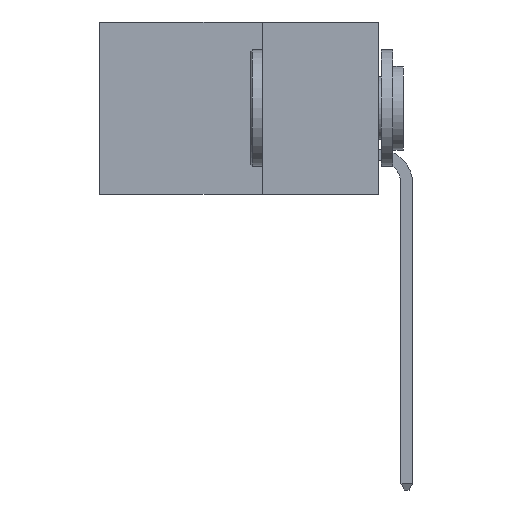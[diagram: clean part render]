
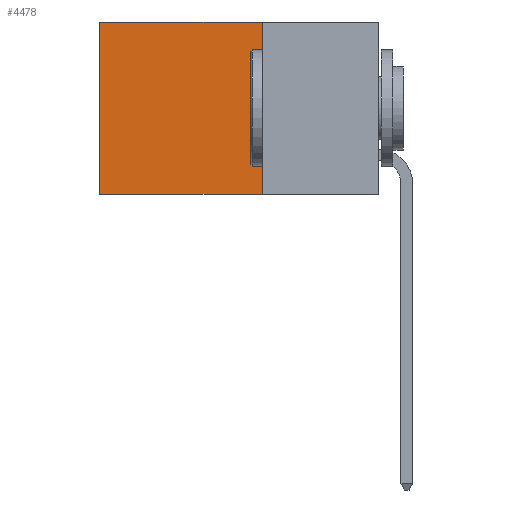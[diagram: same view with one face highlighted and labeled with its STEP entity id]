
A CAD part, left-side view. The second image highlights one B-rep face of the part: STEP entity #4478.
In plain terms, the highlighted planar face has unit normal (-1, 0, 0).
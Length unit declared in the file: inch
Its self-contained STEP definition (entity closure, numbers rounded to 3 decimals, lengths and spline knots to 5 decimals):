
#2251 = EDGE_CURVE ( 'NONE', #13459, #15585, #3702, .T. ) ;
#2489 = LINE ( 'NONE', #6536, #6465 ) ;
#3702 = LINE ( 'NONE', #6270, #20454 ) ;
#4478 = ADVANCED_FACE ( 'NONE', ( #19866 ), #14140, .F. ) ;
#5267 = DIRECTION ( 'NONE',  ( 0., 0., -1. ) ) ;
#6270 = CARTESIAN_POINT ( 'NONE',  ( 0.2615, 0.25, -0.37 ) ) ;
#6465 = VECTOR ( 'NONE', #5267, 39.37008 ) ;
#6536 = CARTESIAN_POINT ( 'NONE',  ( 0.2615, 0.6, -0.37 ) ) ;
#7289 = CARTESIAN_POINT ( 'NONE',  ( 0.2615, 0.6, -0.37 ) ) ;
#7563 = DIRECTION ( 'NONE',  ( 0., 1., 0. ) ) ;
#7832 = ORIENTED_EDGE ( 'NONE', *, *, #8437, .F. ) ;
#8437 = EDGE_CURVE ( 'NONE', #11577, #13459, #15739, .T. ) ;
#8834 = EDGE_CURVE ( 'NONE', #11577, #19460, #11801, .T. ) ;
#9093 = EDGE_CURVE ( 'NONE', #19460, #15585, #2489, .T. ) ;
#10314 = CARTESIAN_POINT ( 'NONE',  ( 0.2615, 0.25, -0.37 ) ) ;
#10750 = VECTOR ( 'NONE', #20789, 39.37008 ) ;
#11440 = DIRECTION ( 'NONE',  ( 0., 1., 0. ) ) ;
#11494 = CARTESIAN_POINT ( 'NONE',  ( 0.2615, 0.25, 0. ) ) ;
#11562 = ORIENTED_EDGE ( 'NONE', *, *, #8834, .T. ) ;
#11577 = VERTEX_POINT ( 'NONE', #13075 ) ;
#11801 = LINE ( 'NONE', #11494, #12315 ) ;
#12047 = ORIENTED_EDGE ( 'NONE', *, *, #9093, .T. ) ;
#12315 = VECTOR ( 'NONE', #11440, 39.37008 ) ;
#13075 = CARTESIAN_POINT ( 'NONE',  ( 0.2615, 0.25, 0. ) ) ;
#13459 = VERTEX_POINT ( 'NONE', #10314 ) ;
#13947 = DIRECTION ( 'NONE',  ( 0., 0., -1. ) ) ;
#13950 = DIRECTION ( 'NONE',  ( 1., 0., 0. ) ) ;
#14037 = EDGE_LOOP ( 'NONE', ( #12047, #17597, #7832, #11562 ) ) ;
#14140 = PLANE ( 'NONE',  #18800 ) ;
#14210 = CARTESIAN_POINT ( 'NONE',  ( 0.2615, 0.25, -0.37 ) ) ;
#15585 = VERTEX_POINT ( 'NONE', #7289 ) ;
#15739 = LINE ( 'NONE', #21401, #10750 ) ;
#17597 = ORIENTED_EDGE ( 'NONE', *, *, #2251, .F. ) ;
#18800 = AXIS2_PLACEMENT_3D ( 'NONE', #14210, #13950, #13947 ) ;
#19460 = VERTEX_POINT ( 'NONE', #21373 ) ;
#19866 = FACE_OUTER_BOUND ( 'NONE', #14037, .T. ) ;
#20454 = VECTOR ( 'NONE', #7563, 39.37008 ) ;
#20789 = DIRECTION ( 'NONE',  ( 0., 0., -1. ) ) ;
#21373 = CARTESIAN_POINT ( 'NONE',  ( 0.2615, 0.6, 0. ) ) ;
#21401 = CARTESIAN_POINT ( 'NONE',  ( 0.2615, 0.25, -0.37 ) ) ;
